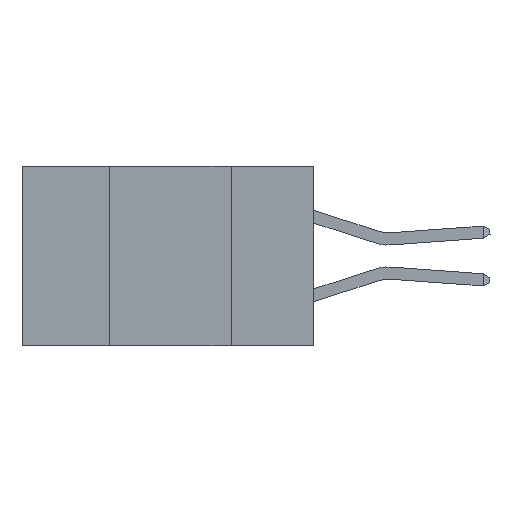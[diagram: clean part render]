
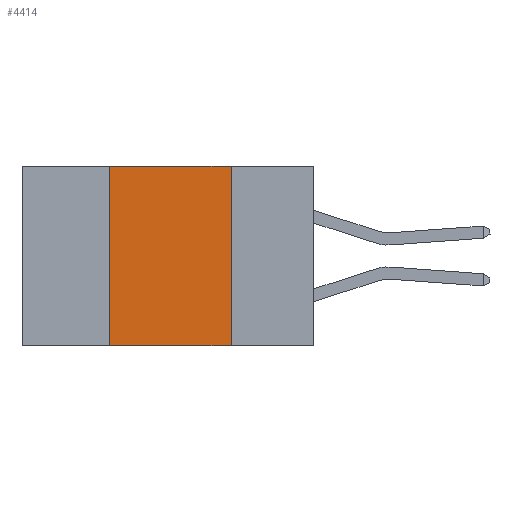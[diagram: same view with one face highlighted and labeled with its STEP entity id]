
A CAD part, left-side view. The second image highlights one B-rep face of the part: STEP entity #4414.
In plain terms, the highlighted planar face has unit normal (-1, 0, 0).
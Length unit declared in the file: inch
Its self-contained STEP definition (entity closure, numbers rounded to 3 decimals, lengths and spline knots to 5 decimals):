
#251 = CARTESIAN_POINT ( 'NONE',  ( 0., 0.17, 0. ) ) ;
#992 = VERTEX_POINT ( 'NONE', #18880 ) ;
#1026 = ORIENTED_EDGE ( 'NONE', *, *, #4574, .F. ) ;
#2326 = LINE ( 'NONE', #3310, #9616 ) ;
#2992 = CARTESIAN_POINT ( 'NONE',  ( 0., 0.42, 0. ) ) ;
#3310 = CARTESIAN_POINT ( 'NONE',  ( 0., 0.17, 0. ) ) ;
#4414 = ADVANCED_FACE ( 'NONE', ( #13364 ), #17137, .F. ) ;
#4574 = EDGE_CURVE ( 'NONE', #992, #13539, #10387, .T. ) ;
#5681 = LINE ( 'NONE', #2992, #16920 ) ;
#5904 = VECTOR ( 'NONE', #9163, 39.37008 ) ;
#8194 = DIRECTION ( 'NONE',  ( 0., 0., -1. ) ) ;
#8981 = DIRECTION ( 'NONE',  ( 0., -1., 0. ) ) ;
#9163 = DIRECTION ( 'NONE',  ( 0., -1., 0. ) ) ;
#9616 = VECTOR ( 'NONE', #8194, 39.37008 ) ;
#9945 = VECTOR ( 'NONE', #8981, 39.37008 ) ;
#10384 = EDGE_CURVE ( 'NONE', #14617, #19586, #11449, .T. ) ;
#10387 = LINE ( 'NONE', #17114, #5904 ) ;
#10709 = DIRECTION ( 'NONE',  ( 1., 0., 0. ) ) ;
#10913 = CARTESIAN_POINT ( 'NONE',  ( 0., 0.6, 0. ) ) ;
#11052 = ORIENTED_EDGE ( 'NONE', *, *, #11248, .F. ) ;
#11248 = EDGE_CURVE ( 'NONE', #14617, #992, #5681, .T. ) ;
#11449 = LINE ( 'NONE', #20135, #9945 ) ;
#12438 = DIRECTION ( 'NONE',  ( 0., 0., 1. ) ) ;
#13364 = FACE_OUTER_BOUND ( 'NONE', #18808, .T. ) ;
#13539 = VERTEX_POINT ( 'NONE', #251 ) ;
#14061 = AXIS2_PLACEMENT_3D ( 'NONE', #10913, #10709, #20331 ) ;
#14617 = VERTEX_POINT ( 'NONE', #15772 ) ;
#15390 = EDGE_CURVE ( 'NONE', #13539, #19586, #2326, .T. ) ;
#15772 = CARTESIAN_POINT ( 'NONE',  ( 0., 0.42, -0.37 ) ) ;
#16920 = VECTOR ( 'NONE', #12438, 39.37008 ) ;
#17114 = CARTESIAN_POINT ( 'NONE',  ( 0., 0.6, 0. ) ) ;
#17137 = PLANE ( 'NONE',  #14061 ) ;
#17419 = ORIENTED_EDGE ( 'NONE', *, *, #10384, .T. ) ;
#18684 = ORIENTED_EDGE ( 'NONE', *, *, #15390, .F. ) ;
#18808 = EDGE_LOOP ( 'NONE', ( #18684, #1026, #11052, #17419 ) ) ;
#18880 = CARTESIAN_POINT ( 'NONE',  ( 0., 0.42, 0. ) ) ;
#19586 = VERTEX_POINT ( 'NONE', #20419 ) ;
#20135 = CARTESIAN_POINT ( 'NONE',  ( 0., 0.6, -0.37 ) ) ;
#20331 = DIRECTION ( 'NONE',  ( 0., 0., -1. ) ) ;
#20419 = CARTESIAN_POINT ( 'NONE',  ( 0., 0.17, -0.37 ) ) ;
